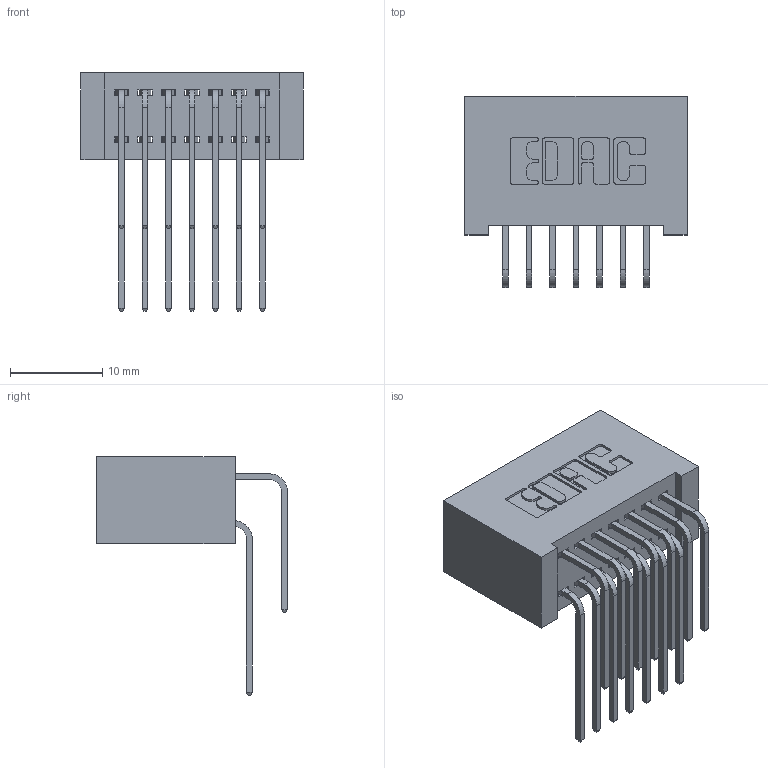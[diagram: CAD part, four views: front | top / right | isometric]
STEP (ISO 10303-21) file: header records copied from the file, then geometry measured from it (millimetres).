
FILE_DESCRIPTION (( 'STEP AP203' ), '1' );
FILE_NAME ('342-014-559-201.STEP', '2018-08-10T18:38:25', ( '' ), ( '' ), 'SwSTEP 2.0', 'SolidWorks 2016', '' );
FILE_SCHEMA (( 'CONFIG_CONTROL_DESIGN' ));
Length unit declared in the file: inch
Products named in the file (4): 342-014-559-201; 342 Part_Lugless; 345-292-001_558 559 Tail - 1; 345-292-001_559 Tail - 2
Assembly tree (15 placements, depth 2):
  342-014-559-201
    342 Part_Lugless
    345-292-001_558 559 Tail - 1  x7
    345-292-001_559 Tail - 2  x7
Bounding box: 24.03 x 20.64 x 25.78 mm (x, y, z)
Volume: 2513.6 mm3; surface area: 4040.6 mm2
Topology: 15 solids, 15 shells, 858 faces, 2529 edges, 1666 vertices
Faces by surface type: plane 594, cylinder 264
Entity records: 10405 total; most frequent: CARTESIAN_POINT 1813, ORIENTED_EDGE 1698, DIRECTION 1585, EDGE_CURVE 849, LINE 689, VECTOR 689, VERTEX_POINT 562, AXIS2_PLACEMENT_3D 448
